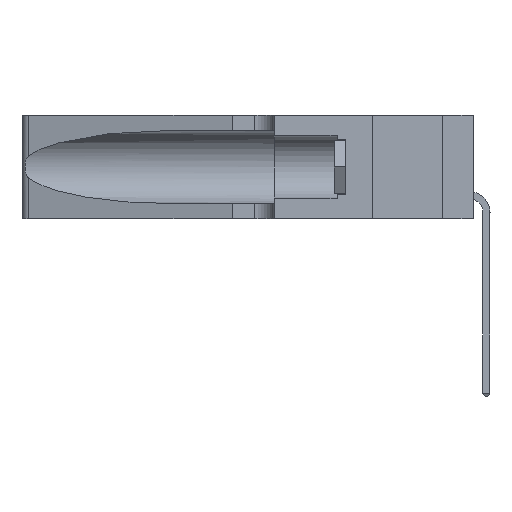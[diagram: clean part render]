
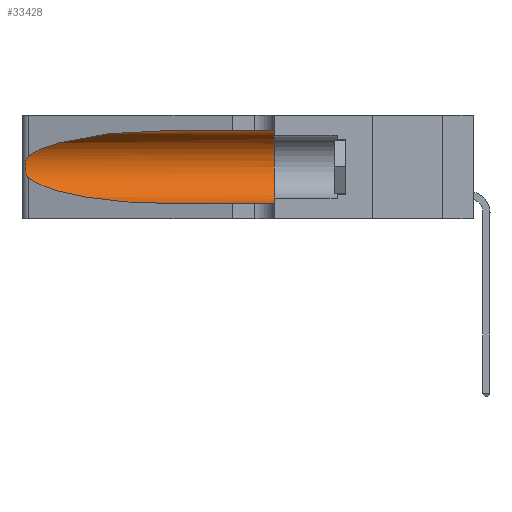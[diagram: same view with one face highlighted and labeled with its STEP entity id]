
A CAD part, left-side view. The second image highlights one B-rep face of the part: STEP entity #33428.
In plain terms, the highlighted cylindrical face has radius 3.308 mm (diameter 6.617 mm), a partial arc.
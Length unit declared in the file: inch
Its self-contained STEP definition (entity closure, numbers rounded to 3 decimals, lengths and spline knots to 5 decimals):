
#865 = CARTESIAN_POINT ( 'NONE',  ( 0.25487, 1.22718, 0.22369 ) ) ;
#913 = CARTESIAN_POINT ( 'NONE',  ( 0.25555, 1.22994, 0.2215 ) ) ;
#1057 = LINE ( 'NONE', #14928, #34362 ) ;
#1086 = CARTESIAN_POINT ( 'NONE',  ( 0.25854, 1.2359, 0.20912 ) ) ;
#3635 = ORIENTED_EDGE ( 'NONE', *, *, #26728, .T. ) ;
#3762 = DIRECTION ( 'NONE',  ( 0., 1., 0. ) ) ;
#4091 = ORIENTED_EDGE ( 'NONE', *, *, #10548, .F. ) ;
#4181 = CARTESIAN_POINT ( 'NONE',  ( 0.25789, 1.23486, 0.15765 ) ) ;
#6035 = CARTESIAN_POINT ( 'NONE',  ( 0.25487, 1.22718, 0.14631 ) ) ;
#7069 = CARTESIAN_POINT ( 'NONE',  ( 0.2373, 1.15595, 0.28018 ) ) ;
#7632 = DIRECTION ( 'NONE',  ( 0., 0., 1. ) ) ;
#7964 = VERTEX_POINT ( 'NONE', #34368 ) ;
#8082 = AXIS2_PLACEMENT_3D ( 'NONE', #22277, #3762, #7632 ) ;
#8178 = FACE_OUTER_BOUND ( 'NONE', #38100, .T. ) ;
#8356 = CARTESIAN_POINT ( 'NONE',  ( 0.25639, 1.23186, 0.15144 ) ) ;
#8520 = CARTESIAN_POINT ( 'NONE',  ( 0.25555, 1.22993, 0.14849 ) ) ;
#8922 = ORIENTED_EDGE ( 'NONE', *, *, #17545, .T. ) ;
#8991 = CARTESIAN_POINT ( 'NONE',  ( 0.1305, 0.35, 0.05475 ) ) ;
#10548 = EDGE_CURVE ( 'NONE', #37570, #43225, #1057, .T. ) ;
#12002 = DIRECTION ( 'NONE',  ( 0., -1., 0. ) ) ;
#12759 = LINE ( 'NONE', #38445, #26017 ) ;
#12860 = EDGE_CURVE ( 'NONE', #43225, #22331, #46262, .T. ) ;
#14771 = CARTESIAN_POINT ( 'NONE',  ( 0.25487, 1.22718, 0.22369 ) ) ;
#14928 = CARTESIAN_POINT ( 'NONE',  ( 0.1305, 1.61858, 0.31525 ) ) ;
#16469 = DIRECTION ( 'NONE',  ( 0., -1., 0. ) ) ;
#16520 = DIRECTION ( 'NONE',  ( 0., 0., -1. ) ) ;
#17545 = EDGE_CURVE ( 'NONE', #37570, #37032, #24884, .T. ) ;
#17646 = CARTESIAN_POINT ( 'NONE',  ( 0.1305, 1.61858, 0.185 ) ) ;
#18834 = CARTESIAN_POINT ( 'NONE',  ( 0.25487, 1.22718, 0.14631 ) ) ;
#18867 = CARTESIAN_POINT ( 'NONE',  ( 0.1305, 0.35, 0.31525 ) ) ;
#18986 = CARTESIAN_POINT ( 'NONE',  ( 0.26075, 1.23896, 0.178 ) ) ;
#21336 = B_SPLINE_CURVE_WITH_KNOTS ( 'NONE', 3,
 ( #33973, #913, #22543, #23010, #1086, #33663, #41031, #18986, #26826, #41358, #4181, #8356, #8520, #18834 ),
 .UNSPECIFIED., .F., .F.,
 ( 4, 2, 2, 2, 2, 2, 4 ),
 ( 0., 0.00027, 0.00053, 0.00107, 0.0016, 0.00187, 0.00214 ),
 .UNSPECIFIED. ) ;
#21724 = CARTESIAN_POINT ( 'NONE',  ( 0.1305, 0.72297, 0.31525 ) ) ;
#22193 = EDGE_CURVE ( 'NONE', #37032, #35289, #21336, .T. ) ;
#22277 = CARTESIAN_POINT ( 'NONE',  ( 0.1305, 0.35, 0.185 ) ) ;
#22331 = VERTEX_POINT ( 'NONE', #8991 ) ;
#22543 = CARTESIAN_POINT ( 'NONE',  ( 0.25639, 1.23184, 0.21858 ) ) ;
#22613 = ORIENTED_EDGE ( 'NONE', *, *, #12860, .F. ) ;
#23010 = CARTESIAN_POINT ( 'NONE',  ( 0.25787, 1.23484, 0.2124 ) ) ;
#24121 = CARTESIAN_POINT ( 'NONE',  ( 0.2373, 1.15595, 0.08982 ) ) ;
#24884 =( BOUNDED_CURVE ( )  B_SPLINE_CURVE ( 3, ( #21724, #43945, #7069, #14771 ),
 .UNSPECIFIED., .F., .T. ) 
 B_SPLINE_CURVE_WITH_KNOTS ( ( 4, 4 ),
 ( 1.5708, 2.84003 ),
 .UNSPECIFIED. ) 
 CURVE ( )  GEOMETRIC_REPRESENTATION_ITEM ( )  RATIONAL_B_SPLINE_CURVE ( ( 1., 0.87, 0.87, 1. ) ) 
 REPRESENTATION_ITEM ( '' )  );
#26017 = VECTOR ( 'NONE', #16469, 39.37008 ) ;
#26728 = EDGE_CURVE ( 'NONE', #35289, #7964, #36286, .T. ) ;
#26826 = CARTESIAN_POINT ( 'NONE',  ( 0.26017, 1.23833, 0.17102 ) ) ;
#28233 = CYLINDRICAL_SURFACE ( 'NONE', #31952, 0.13025 ) ;
#28360 = CARTESIAN_POINT ( 'NONE',  ( 0.1305, 0.72297, 0.05475 ) ) ;
#30020 = ORIENTED_EDGE ( 'NONE', *, *, #22193, .T. ) ;
#31952 = AXIS2_PLACEMENT_3D ( 'NONE', #17646, #35059, #16520 ) ;
#33267 = EDGE_CURVE ( 'NONE', #7964, #22331, #12759, .T. ) ;
#33428 = ADVANCED_FACE ( 'NONE', ( #8178 ), #28233, .F. ) ;
#33663 = CARTESIAN_POINT ( 'NONE',  ( 0.26018, 1.23835, 0.19895 ) ) ;
#33973 = CARTESIAN_POINT ( 'NONE',  ( 0.25487, 1.22718, 0.22369 ) ) ;
#34362 = VECTOR ( 'NONE', #12002, 39.37008 ) ;
#34368 = CARTESIAN_POINT ( 'NONE',  ( 0.1305, 0.72297, 0.05475 ) ) ;
#34538 = CARTESIAN_POINT ( 'NONE',  ( 0.1305, 0.72297, 0.31525 ) ) ;
#35059 = DIRECTION ( 'NONE',  ( 0., -1., 0. ) ) ;
#35289 = VERTEX_POINT ( 'NONE', #6035 ) ;
#36286 =( BOUNDED_CURVE ( )  B_SPLINE_CURVE ( 3, ( #42616, #24121, #38956, #28360 ),
 .UNSPECIFIED., .F., .T. ) 
 B_SPLINE_CURVE_WITH_KNOTS ( ( 4, 4 ),
 ( 3.44316, 4.71239 ),
 .UNSPECIFIED. ) 
 CURVE ( )  GEOMETRIC_REPRESENTATION_ITEM ( )  RATIONAL_B_SPLINE_CURVE ( ( 1., 0.87, 0.87, 1. ) ) 
 REPRESENTATION_ITEM ( '' )  );
#37032 = VERTEX_POINT ( 'NONE', #865 ) ;
#37570 = VERTEX_POINT ( 'NONE', #34538 ) ;
#38100 = EDGE_LOOP ( 'NONE', ( #8922, #30020, #3635, #40200, #22613, #4091 ) ) ;
#38445 = CARTESIAN_POINT ( 'NONE',  ( 0.1305, 1.61858, 0.05475 ) ) ;
#38956 = CARTESIAN_POINT ( 'NONE',  ( 0.18966, 0.96281, 0.05475 ) ) ;
#40200 = ORIENTED_EDGE ( 'NONE', *, *, #33267, .T. ) ;
#41031 = CARTESIAN_POINT ( 'NONE',  ( 0.26075, 1.23896, 0.19203 ) ) ;
#41358 = CARTESIAN_POINT ( 'NONE',  ( 0.25856, 1.23593, 0.16098 ) ) ;
#42616 = CARTESIAN_POINT ( 'NONE',  ( 0.25487, 1.22718, 0.14631 ) ) ;
#43225 = VERTEX_POINT ( 'NONE', #18867 ) ;
#43945 = CARTESIAN_POINT ( 'NONE',  ( 0.18966, 0.96281, 0.31525 ) ) ;
#46262 = CIRCLE ( 'NONE', #8082, 0.13025 ) ;
